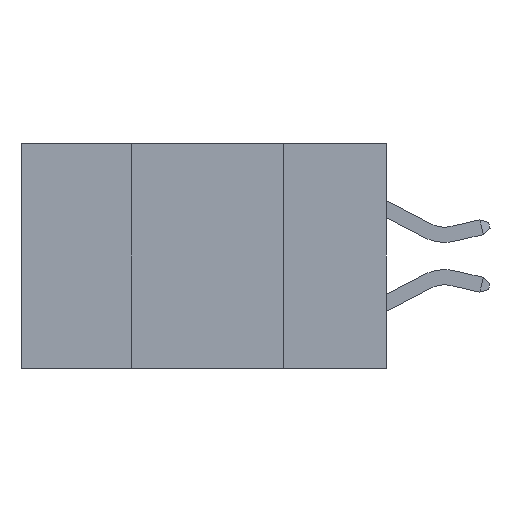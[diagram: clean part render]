
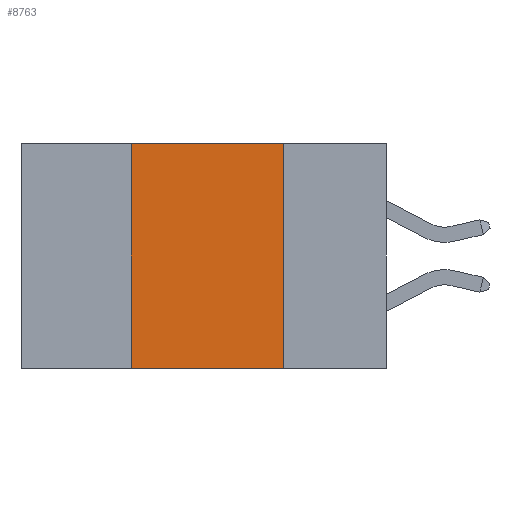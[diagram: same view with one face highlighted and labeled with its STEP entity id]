
A CAD part, left-side view. The second image highlights one B-rep face of the part: STEP entity #8763.
In plain terms, the highlighted planar face has unit normal (-1, 0, 0).
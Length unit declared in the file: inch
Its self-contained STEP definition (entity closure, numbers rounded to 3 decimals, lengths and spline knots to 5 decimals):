
#214 = CARTESIAN_POINT ( 'NONE',  ( 0., 0.17, 0. ) ) ;
#2358 = CARTESIAN_POINT ( 'NONE',  ( 0., 0.42, 0. ) ) ;
#2596 = CARTESIAN_POINT ( 'NONE',  ( 0., 0.17, -0.37 ) ) ;
#3274 = VERTEX_POINT ( 'NONE', #214 ) ;
#3656 = ORIENTED_EDGE ( 'NONE', *, *, #21890, .F. ) ;
#7447 = EDGE_CURVE ( 'NONE', #8818, #22218, #22372, .T. ) ;
#8763 = ADVANCED_FACE ( 'NONE', ( #11895 ), #26234, .F. ) ;
#8818 = VERTEX_POINT ( 'NONE', #19115 ) ;
#8902 = DIRECTION ( 'NONE',  ( 0., 0., -1. ) ) ;
#8917 = EDGE_CURVE ( 'NONE', #19641, #3274, #21126, .T. ) ;
#11175 = VECTOR ( 'NONE', #13289, 39.37008 ) ;
#11770 = CARTESIAN_POINT ( 'NONE',  ( 0., 0.6, 0. ) ) ;
#11893 = DIRECTION ( 'NONE',  ( 0., -1., 0. ) ) ;
#11895 = FACE_OUTER_BOUND ( 'NONE', #22798, .T. ) ;
#12699 = CARTESIAN_POINT ( 'NONE',  ( 0., 0.17, -0.37 ) ) ;
#12740 = CARTESIAN_POINT ( 'NONE',  ( 0., 0.42, -0.37 ) ) ;
#13289 = DIRECTION ( 'NONE',  ( 0., 0., 1. ) ) ;
#14166 = EDGE_CURVE ( 'NONE', #8818, #19641, #16825, .T. ) ;
#14817 = VECTOR ( 'NONE', #8902, 39.37008 ) ;
#15004 = LINE ( 'NONE', #12699, #14817 ) ;
#15845 = DIRECTION ( 'NONE',  ( 1., 0., 0. ) ) ;
#16234 = DIRECTION ( 'NONE',  ( 0., 0., -1. ) ) ;
#16388 = ORIENTED_EDGE ( 'NONE', *, *, #14166, .F. ) ;
#16634 = DIRECTION ( 'NONE',  ( 0., -1., 0. ) ) ;
#16825 = LINE ( 'NONE', #12740, #11175 ) ;
#18706 = CARTESIAN_POINT ( 'NONE',  ( 0., 0.6, 0. ) ) ;
#19115 = CARTESIAN_POINT ( 'NONE',  ( 0., 0.42, -0.37 ) ) ;
#19641 = VERTEX_POINT ( 'NONE', #2358 ) ;
#21126 = LINE ( 'NONE', #18706, #21644 ) ;
#21162 = AXIS2_PLACEMENT_3D ( 'NONE', #11770, #15845, #16234 ) ;
#21644 = VECTOR ( 'NONE', #16634, 39.37008 ) ;
#21811 = ORIENTED_EDGE ( 'NONE', *, *, #8917, .F. ) ;
#21890 = EDGE_CURVE ( 'NONE', #3274, #22218, #15004, .T. ) ;
#22218 = VERTEX_POINT ( 'NONE', #2596 ) ;
#22246 = CARTESIAN_POINT ( 'NONE',  ( 0., 0.6, -0.37 ) ) ;
#22311 = ORIENTED_EDGE ( 'NONE', *, *, #7447, .T. ) ;
#22372 = LINE ( 'NONE', #22246, #26083 ) ;
#22798 = EDGE_LOOP ( 'NONE', ( #3656, #21811, #16388, #22311 ) ) ;
#26083 = VECTOR ( 'NONE', #11893, 39.37008 ) ;
#26234 = PLANE ( 'NONE',  #21162 ) ;
